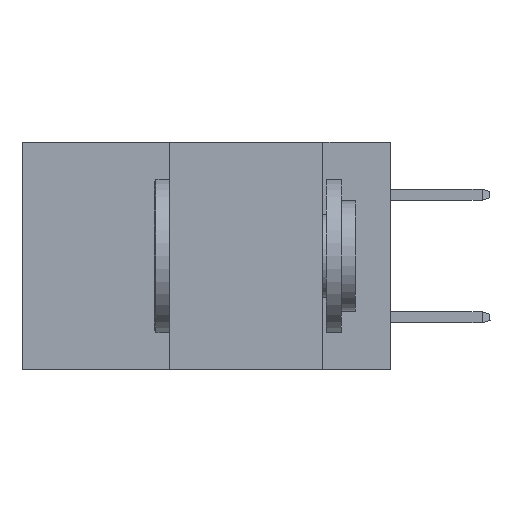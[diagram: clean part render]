
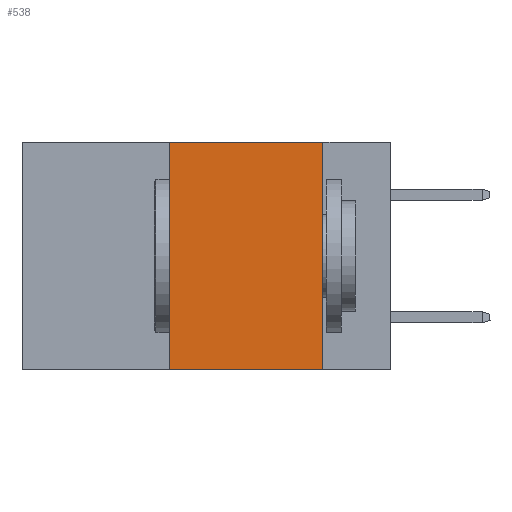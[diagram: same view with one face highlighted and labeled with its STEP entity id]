
A CAD part, left-side view. The second image highlights one B-rep face of the part: STEP entity #538.
In plain terms, the highlighted planar face has unit normal (-1, 0, 0).
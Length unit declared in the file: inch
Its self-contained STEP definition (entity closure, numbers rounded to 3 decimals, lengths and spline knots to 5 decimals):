
#538 = ADVANCED_FACE ( 'NONE', ( #7332 ), #10288, .F. ) ;
#699 = VERTEX_POINT ( 'NONE', #8572 ) ;
#1144 = EDGE_LOOP ( 'NONE', ( #22768, #22575, #1535, #10401 ) ) ;
#1535 = ORIENTED_EDGE ( 'NONE', *, *, #18243, .F. ) ;
#3212 = DIRECTION ( 'NONE',  ( 0., -1., 0. ) ) ;
#4017 = LINE ( 'NONE', #21054, #9666 ) ;
#6170 = VERTEX_POINT ( 'NONE', #23958 ) ;
#6248 = CARTESIAN_POINT ( 'NONE',  ( 0., 0.11, 0. ) ) ;
#6285 = LINE ( 'NONE', #6248, #7484 ) ;
#6678 = CARTESIAN_POINT ( 'NONE',  ( 0., 0.36, 0. ) ) ;
#7332 = FACE_OUTER_BOUND ( 'NONE', #1144, .T. ) ;
#7484 = VECTOR ( 'NONE', #26374, 39.37008 ) ;
#8572 = CARTESIAN_POINT ( 'NONE',  ( 0., 0.36, -0.37 ) ) ;
#9614 = VECTOR ( 'NONE', #11944, 39.37008 ) ;
#9666 = VECTOR ( 'NONE', #11100, 39.37008 ) ;
#10288 = PLANE ( 'NONE',  #15771 ) ;
#10401 = ORIENTED_EDGE ( 'NONE', *, *, #29407, .T. ) ;
#11100 = DIRECTION ( 'NONE',  ( 0., -1., 0. ) ) ;
#11944 = DIRECTION ( 'NONE',  ( 0., 0., 1. ) ) ;
#12855 = DIRECTION ( 'NONE',  ( 1., 0., 0. ) ) ;
#15771 = AXIS2_PLACEMENT_3D ( 'NONE', #20446, #12855, #23146 ) ;
#18094 = VERTEX_POINT ( 'NONE', #21458 ) ;
#18243 = EDGE_CURVE ( 'NONE', #699, #31491, #19624, .T. ) ;
#18745 = EDGE_CURVE ( 'NONE', #31491, #6170, #32765, .T. ) ;
#19624 = LINE ( 'NONE', #6678, #9614 ) ;
#20115 = EDGE_CURVE ( 'NONE', #6170, #18094, #6285, .T. ) ;
#20446 = CARTESIAN_POINT ( 'NONE',  ( 0., 0.6, 0. ) ) ;
#21054 = CARTESIAN_POINT ( 'NONE',  ( 0., 0.6, -0.37 ) ) ;
#21458 = CARTESIAN_POINT ( 'NONE',  ( 0., 0.11, -0.37 ) ) ;
#22575 = ORIENTED_EDGE ( 'NONE', *, *, #18745, .F. ) ;
#22768 = ORIENTED_EDGE ( 'NONE', *, *, #20115, .F. ) ;
#23146 = DIRECTION ( 'NONE',  ( 0., 0., -1. ) ) ;
#23459 = CARTESIAN_POINT ( 'NONE',  ( 0., 0.36, 0. ) ) ;
#23958 = CARTESIAN_POINT ( 'NONE',  ( 0., 0.11, 0. ) ) ;
#26374 = DIRECTION ( 'NONE',  ( 0., 0., -1. ) ) ;
#28026 = VECTOR ( 'NONE', #3212, 39.37008 ) ;
#28986 = CARTESIAN_POINT ( 'NONE',  ( 0., 0.6, 0. ) ) ;
#29407 = EDGE_CURVE ( 'NONE', #699, #18094, #4017, .T. ) ;
#31491 = VERTEX_POINT ( 'NONE', #23459 ) ;
#32765 = LINE ( 'NONE', #28986, #28026 ) ;
